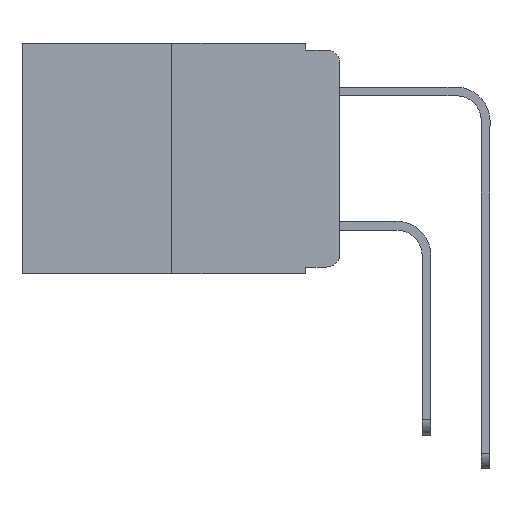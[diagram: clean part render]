
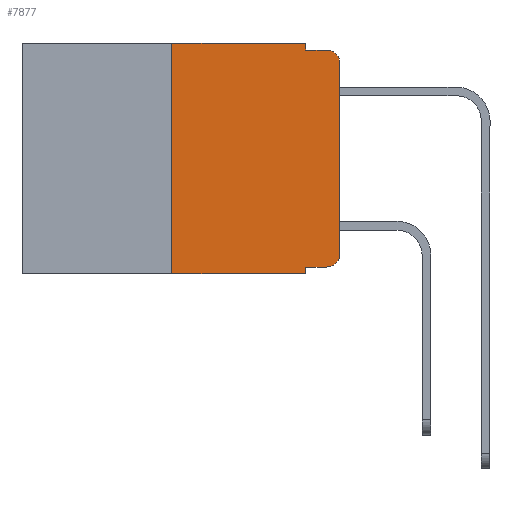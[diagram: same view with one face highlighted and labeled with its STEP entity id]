
A CAD part, left-side view. The second image highlights one B-rep face of the part: STEP entity #7877.
In plain terms, the highlighted planar face has unit normal (-1, 0, 0).
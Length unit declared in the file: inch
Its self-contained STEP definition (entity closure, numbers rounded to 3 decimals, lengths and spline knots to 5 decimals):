
#282 = VERTEX_POINT ( 'NONE', #8029 ) ;
#749 = DIRECTION ( 'NONE',  ( 0., -1., 0. ) ) ;
#875 = CARTESIAN_POINT ( 'NONE',  ( 0., 0.051, -0.333 ) ) ;
#1167 = DIRECTION ( 'NONE',  ( 1., 0., 0. ) ) ;
#1301 = DIRECTION ( 'NONE',  ( 0., 0., -1. ) ) ;
#1392 = EDGE_CURVE ( 'NONE', #2154, #8046, #14046, .T. ) ;
#1775 = CARTESIAN_POINT ( 'NONE',  ( 0., 0., 0. ) ) ;
#1982 = DIRECTION ( 'NONE',  ( 0., -1., 0. ) ) ;
#2095 = LINE ( 'NONE', #8503, #14438 ) ;
#2154 = VERTEX_POINT ( 'NONE', #3462 ) ;
#2307 = EDGE_CURVE ( 'NONE', #14133, #2154, #12402, .T. ) ;
#2391 = ORIENTED_EDGE ( 'NONE', *, *, #9440, .F. ) ;
#2777 = VECTOR ( 'NONE', #4355, 39.37008 ) ;
#2800 = ORIENTED_EDGE ( 'NONE', *, *, #3161, .F. ) ;
#3073 = VECTOR ( 'NONE', #749, 39.37008 ) ;
#3161 = EDGE_CURVE ( 'NONE', #14133, #14013, #2095, .T. ) ;
#3202 = DIRECTION ( 'NONE',  ( 0., 0., -1. ) ) ;
#3462 = CARTESIAN_POINT ( 'NONE',  ( 0., 0.02, -0.333 ) ) ;
#3538 = CARTESIAN_POINT ( 'NONE',  ( 0., 0.051, -0.343 ) ) ;
#3795 = VECTOR ( 'NONE', #13734, 39.37008 ) ;
#4355 = DIRECTION ( 'NONE',  ( 0., -1., 0. ) ) ;
#4435 = DIRECTION ( 'NONE',  ( 0., 0., 1. ) ) ;
#4444 = VERTEX_POINT ( 'NONE', #15415 ) ;
#4599 = LINE ( 'NONE', #10285, #3795 ) ;
#4841 = AXIS2_PLACEMENT_3D ( 'NONE', #5069, #1167, #9940 ) ;
#5069 = CARTESIAN_POINT ( 'NONE',  ( 0., 0.473, 0. ) ) ;
#5256 = CARTESIAN_POINT ( 'NONE',  ( 0., 0.051, 0. ) ) ;
#5459 = ORIENTED_EDGE ( 'NONE', *, *, #9031, .F. ) ;
#6221 = LINE ( 'NONE', #6859, #2777 ) ;
#6280 = LINE ( 'NONE', #1775, #9101 ) ;
#6541 = DIRECTION ( 'NONE',  ( 0., 0., -1. ) ) ;
#6680 = VERTEX_POINT ( 'NONE', #14752 ) ;
#6778 = FACE_OUTER_BOUND ( 'NONE', #12104, .T. ) ;
#6846 = EDGE_CURVE ( 'NONE', #282, #14013, #6221, .T. ) ;
#6859 = CARTESIAN_POINT ( 'NONE',  ( 0., 0.473, -0.343 ) ) ;
#6901 = VERTEX_POINT ( 'NONE', #13948 ) ;
#7462 = EDGE_CURVE ( 'NONE', #282, #13273, #4599, .T. ) ;
#7877 = ADVANCED_FACE ( 'NONE', ( #6778 ), #8754, .F. ) ;
#7957 = CARTESIAN_POINT ( 'NONE',  ( 0., 0.25, 0. ) ) ;
#8029 = CARTESIAN_POINT ( 'NONE',  ( 0., 0.25, -0.343 ) ) ;
#8046 = VERTEX_POINT ( 'NONE', #15536 ) ;
#8229 = EDGE_CURVE ( 'NONE', #10300, #6901, #11357, .T. ) ;
#8401 = VECTOR ( 'NONE', #1982, 39.37008 ) ;
#8503 = CARTESIAN_POINT ( 'NONE',  ( 0., 0.051, 0. ) ) ;
#8731 = CIRCLE ( 'NONE', #14007, 0.02 ) ;
#8754 = PLANE ( 'NONE',  #4841 ) ;
#8875 = DIRECTION ( 'NONE',  ( -1., 0., 0. ) ) ;
#9031 = EDGE_CURVE ( 'NONE', #6901, #4444, #11883, .T. ) ;
#9101 = VECTOR ( 'NONE', #4435, 39.37008 ) ;
#9435 = ORIENTED_EDGE ( 'NONE', *, *, #2307, .T. ) ;
#9440 = EDGE_CURVE ( 'NONE', #13273, #10300, #14909, .T. ) ;
#9547 = DIRECTION ( 'NONE',  ( 0., -1., 0. ) ) ;
#9940 = DIRECTION ( 'NONE',  ( 0., 0., -1. ) ) ;
#10285 = CARTESIAN_POINT ( 'NONE',  ( 0., 0.25, 0. ) ) ;
#10300 = VERTEX_POINT ( 'NONE', #12405 ) ;
#11357 = LINE ( 'NONE', #5256, #14780 ) ;
#11367 = EDGE_CURVE ( 'NONE', #6680, #4444, #8731, .T. ) ;
#11416 = ORIENTED_EDGE ( 'NONE', *, *, #12150, .T. ) ;
#11514 = VECTOR ( 'NONE', #9547, 39.37008 ) ;
#11883 = LINE ( 'NONE', #15298, #11514 ) ;
#12104 = EDGE_LOOP ( 'NONE', ( #11416, #14492, #5459, #14836, #2391, #12157, #15213, #2800, #9435, #12875 ) ) ;
#12150 = EDGE_CURVE ( 'NONE', #8046, #6680, #6280, .T. ) ;
#12157 = ORIENTED_EDGE ( 'NONE', *, *, #7462, .F. ) ;
#12402 = LINE ( 'NONE', #875, #3073 ) ;
#12405 = CARTESIAN_POINT ( 'NONE',  ( 0., 0.051, 0. ) ) ;
#12875 = ORIENTED_EDGE ( 'NONE', *, *, #1392, .T. ) ;
#13273 = VERTEX_POINT ( 'NONE', #7957 ) ;
#13731 = AXIS2_PLACEMENT_3D ( 'NONE', #14711, #14696, #3202 ) ;
#13734 = DIRECTION ( 'NONE',  ( 0., 0., 1. ) ) ;
#13948 = CARTESIAN_POINT ( 'NONE',  ( 0., 0.051, -0.01 ) ) ;
#14007 = AXIS2_PLACEMENT_3D ( 'NONE', #15800, #8875, #1301 ) ;
#14013 = VERTEX_POINT ( 'NONE', #3538 ) ;
#14046 = CIRCLE ( 'NONE', #13731, 0.02 ) ;
#14133 = VERTEX_POINT ( 'NONE', #15693 ) ;
#14438 = VECTOR ( 'NONE', #14464, 39.37008 ) ;
#14464 = DIRECTION ( 'NONE',  ( 0., 0., -1. ) ) ;
#14492 = ORIENTED_EDGE ( 'NONE', *, *, #11367, .T. ) ;
#14696 = DIRECTION ( 'NONE',  ( -1., 0., 0. ) ) ;
#14711 = CARTESIAN_POINT ( 'NONE',  ( 0., 0.02, -0.313 ) ) ;
#14752 = CARTESIAN_POINT ( 'NONE',  ( 0., 0., -0.03 ) ) ;
#14780 = VECTOR ( 'NONE', #6541, 39.37008 ) ;
#14836 = ORIENTED_EDGE ( 'NONE', *, *, #8229, .F. ) ;
#14909 = LINE ( 'NONE', #15243, #8401 ) ;
#15213 = ORIENTED_EDGE ( 'NONE', *, *, #6846, .T. ) ;
#15243 = CARTESIAN_POINT ( 'NONE',  ( 0., 0.473, 0. ) ) ;
#15298 = CARTESIAN_POINT ( 'NONE',  ( 0., 0.051, -0.01 ) ) ;
#15415 = CARTESIAN_POINT ( 'NONE',  ( 0., 0.02, -0.01 ) ) ;
#15536 = CARTESIAN_POINT ( 'NONE',  ( 0., 0., -0.313 ) ) ;
#15693 = CARTESIAN_POINT ( 'NONE',  ( 0., 0.051, -0.333 ) ) ;
#15800 = CARTESIAN_POINT ( 'NONE',  ( 0., 0.02, -0.03 ) ) ;
